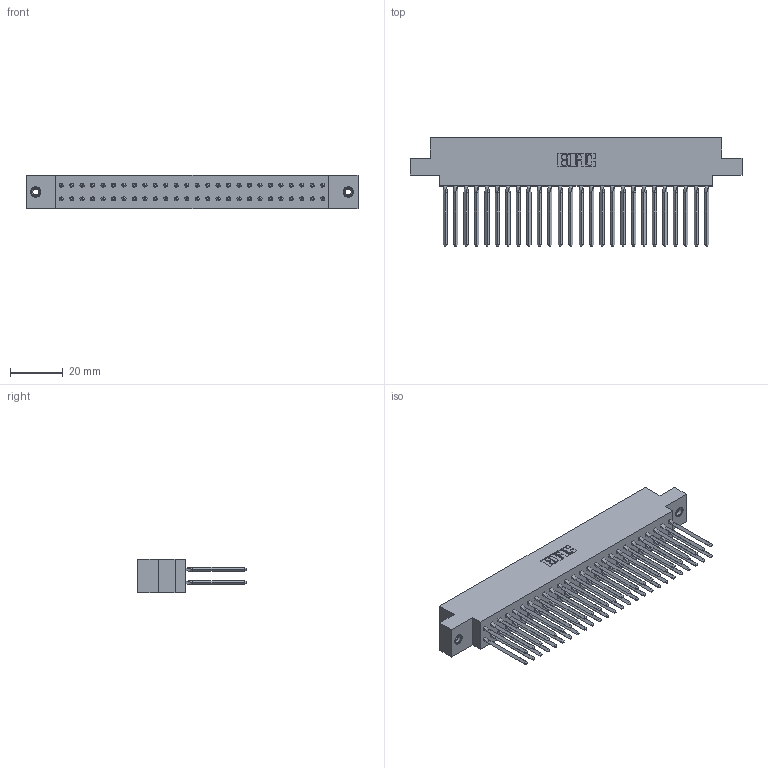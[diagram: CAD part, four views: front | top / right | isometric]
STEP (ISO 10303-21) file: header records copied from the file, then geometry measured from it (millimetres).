
FILE_DESCRIPTION (( 'STEP AP203' ), '1' );
FILE_NAME ('317-052-543-808.STEP', '2020-02-28T03:44:10', ( '' ), ( '' ), 'SwSTEP 2.0', 'SolidWorks 2016', '' );
FILE_SCHEMA (( 'CONFIG_CONTROL_DESIGN' ));
Length unit declared in the file: inch
Products named in the file (4): 345-250-001_345-250-003-102; 317-290-001_543; 317-052-543-808; 317 Part_.156 Dia - TI
Assembly tree (55 placements, depth 2):
  317-052-543-808
    317 Part_.156 Dia - TI
    317-290-001_543  x52
    345-250-001_345-250-003-102  x2
Bounding box: 125.73 x 41.15 x 12.7 mm (x, y, z)
Volume: 20812.7 mm3; surface area: 30967.7 mm2
Topology: 55 solids, 55 shells, 4790 faces, 13255 edges, 8534 vertices
Faces by surface type: plane 3886, cylinder 680, bspline 208, cone 12, torus 4
Entity records: 41001 total; most frequent: CARTESIAN_POINT 7538, ORIENTED_EDGE 7030, DIRECTION 5907, EDGE_CURVE 3515, LINE 3239, VECTOR 3239, VERTEX_POINT 2333, AXIS2_PLACEMENT_3D 1334
